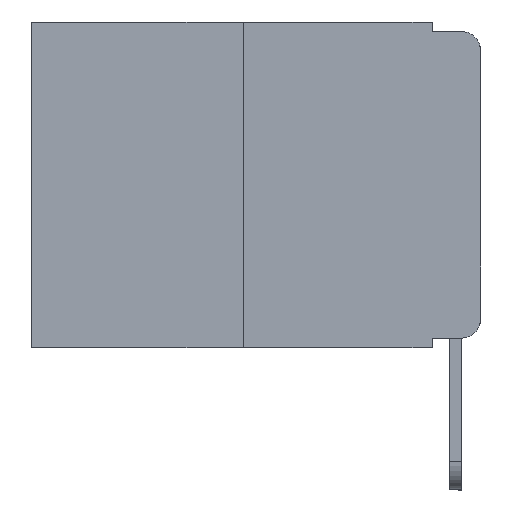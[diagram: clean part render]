
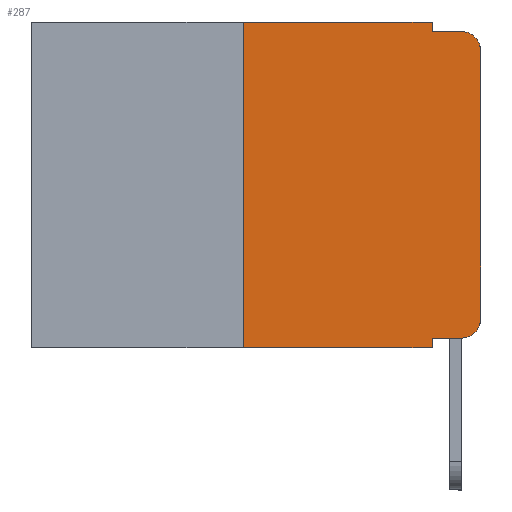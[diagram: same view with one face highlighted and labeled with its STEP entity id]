
A CAD part, left-side view. The second image highlights one B-rep face of the part: STEP entity #287.
In plain terms, the highlighted planar face has unit normal (-1, 0, 0).
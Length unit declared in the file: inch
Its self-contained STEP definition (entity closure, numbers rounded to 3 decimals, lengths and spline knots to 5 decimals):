
#204 = EDGE_CURVE ( 'NONE', #2949, #7871, #11588, .T. ) ;
#226 = VERTEX_POINT ( 'NONE', #18269 ) ;
#287 = ADVANCED_FACE ( 'NONE', ( #17137 ), #6791, .F. ) ;
#504 = ORIENTED_EDGE ( 'NONE', *, *, #10203, .T. ) ;
#596 = DIRECTION ( 'NONE',  ( -1., 0., 0. ) ) ;
#1010 = LINE ( 'NONE', #10817, #20700 ) ;
#1974 = EDGE_CURVE ( 'NONE', #20083, #2949, #19958, .T. ) ;
#2082 = EDGE_CURVE ( 'NONE', #226, #15848, #7178, .T. ) ;
#2559 = CARTESIAN_POINT ( 'NONE',  ( 0., 0.25, 0. ) ) ;
#2949 = VERTEX_POINT ( 'NONE', #16776 ) ;
#3070 = LINE ( 'NONE', #10297, #5269 ) ;
#3171 = DIRECTION ( 'NONE',  ( 0., -1., 0. ) ) ;
#3286 = EDGE_CURVE ( 'NONE', #4948, #20257, #3070, .T. ) ;
#3670 = CIRCLE ( 'NONE', #20002, 0.02 ) ;
#4026 = DIRECTION ( 'NONE',  ( 0., -1., 0. ) ) ;
#4035 = VECTOR ( 'NONE', #14112, 39.37008 ) ;
#4695 = CARTESIAN_POINT ( 'NONE',  ( 0., 0., -0.313 ) ) ;
#4697 = ORIENTED_EDGE ( 'NONE', *, *, #9662, .F. ) ;
#4778 = ORIENTED_EDGE ( 'NONE', *, *, #204, .F. ) ;
#4795 = EDGE_CURVE ( 'NONE', #19974, #226, #14518, .T. ) ;
#4948 = VERTEX_POINT ( 'NONE', #18631 ) ;
#4962 = VECTOR ( 'NONE', #15035, 39.37008 ) ;
#5269 = VECTOR ( 'NONE', #16875, 39.37008 ) ;
#5308 = DIRECTION ( 'NONE',  ( -1., 0., 0. ) ) ;
#6047 = CARTESIAN_POINT ( 'NONE',  ( 0., 0., 0. ) ) ;
#6791 = PLANE ( 'NONE',  #11714 ) ;
#6839 = ORIENTED_EDGE ( 'NONE', *, *, #1974, .F. ) ;
#7023 = VERTEX_POINT ( 'NONE', #7986 ) ;
#7178 = CIRCLE ( 'NONE', #19595, 0.02 ) ;
#7370 = ORIENTED_EDGE ( 'NONE', *, *, #10370, .T. ) ;
#7871 = VERTEX_POINT ( 'NONE', #12731 ) ;
#7986 = CARTESIAN_POINT ( 'NONE',  ( 0., 0.25, -0.343 ) ) ;
#8471 = DIRECTION ( 'NONE',  ( 1., 0., 0. ) ) ;
#9662 = EDGE_CURVE ( 'NONE', #7023, #20083, #17819, .T. ) ;
#9742 = ORIENTED_EDGE ( 'NONE', *, *, #9972, .F. ) ;
#9972 = EDGE_CURVE ( 'NONE', #7871, #15848, #1010, .T. ) ;
#10203 = EDGE_CURVE ( 'NONE', #20768, #19974, #3670, .T. ) ;
#10293 = CARTESIAN_POINT ( 'NONE',  ( 0., 0.02, -0.03 ) ) ;
#10297 = CARTESIAN_POINT ( 'NONE',  ( 0., 0.051, 0. ) ) ;
#10370 = EDGE_CURVE ( 'NONE', #7023, #20257, #12221, .T. ) ;
#10817 = CARTESIAN_POINT ( 'NONE',  ( 0., 0.051, -0.01 ) ) ;
#11588 = LINE ( 'NONE', #18483, #4962 ) ;
#11714 = AXIS2_PLACEMENT_3D ( 'NONE', #19130, #8471, #14023 ) ;
#11982 = DIRECTION ( 'NONE',  ( 0., 0., -1. ) ) ;
#12221 = LINE ( 'NONE', #15659, #4035 ) ;
#12380 = CARTESIAN_POINT ( 'NONE',  ( 0., 0.25, 0. ) ) ;
#12553 = VECTOR ( 'NONE', #16152, 39.37008 ) ;
#12731 = CARTESIAN_POINT ( 'NONE',  ( 0., 0.051, -0.01 ) ) ;
#13058 = ORIENTED_EDGE ( 'NONE', *, *, #4795, .T. ) ;
#13373 = CARTESIAN_POINT ( 'NONE',  ( 0., 0.02, -0.313 ) ) ;
#14023 = DIRECTION ( 'NONE',  ( 0., 0., -1. ) ) ;
#14112 = DIRECTION ( 'NONE',  ( 0., -1., 0. ) ) ;
#14518 = LINE ( 'NONE', #6047, #15546 ) ;
#15035 = DIRECTION ( 'NONE',  ( 0., 0., -1. ) ) ;
#15419 = DIRECTION ( 'NONE',  ( 0., -1., 0. ) ) ;
#15546 = VECTOR ( 'NONE', #19615, 39.37008 ) ;
#15659 = CARTESIAN_POINT ( 'NONE',  ( 0., 0.473, -0.343 ) ) ;
#15848 = VERTEX_POINT ( 'NONE', #20930 ) ;
#16038 = ORIENTED_EDGE ( 'NONE', *, *, #3286, .F. ) ;
#16058 = VECTOR ( 'NONE', #3171, 39.37008 ) ;
#16152 = DIRECTION ( 'NONE',  ( 0., 0., 1. ) ) ;
#16776 = CARTESIAN_POINT ( 'NONE',  ( 0., 0.051, 0. ) ) ;
#16779 = CARTESIAN_POINT ( 'NONE',  ( 0., 0.02, -0.333 ) ) ;
#16875 = DIRECTION ( 'NONE',  ( 0., 0., -1. ) ) ;
#17137 = FACE_OUTER_BOUND ( 'NONE', #20873, .T. ) ;
#17224 = DIRECTION ( 'NONE',  ( 0., 0., -1. ) ) ;
#17505 = ORIENTED_EDGE ( 'NONE', *, *, #2082, .T. ) ;
#17819 = LINE ( 'NONE', #2559, #12553 ) ;
#18269 = CARTESIAN_POINT ( 'NONE',  ( 0., 0., -0.03 ) ) ;
#18483 = CARTESIAN_POINT ( 'NONE',  ( 0., 0.051, 0. ) ) ;
#18631 = CARTESIAN_POINT ( 'NONE',  ( 0., 0.051, -0.333 ) ) ;
#18650 = CARTESIAN_POINT ( 'NONE',  ( 0., 0.473, 0. ) ) ;
#18979 = VECTOR ( 'NONE', #15419, 39.37008 ) ;
#19130 = CARTESIAN_POINT ( 'NONE',  ( 0., 0.473, 0. ) ) ;
#19561 = EDGE_CURVE ( 'NONE', #4948, #20768, #20076, .T. ) ;
#19595 = AXIS2_PLACEMENT_3D ( 'NONE', #10293, #596, #11982 ) ;
#19615 = DIRECTION ( 'NONE',  ( 0., 0., 1. ) ) ;
#19657 = ORIENTED_EDGE ( 'NONE', *, *, #19561, .T. ) ;
#19957 = CARTESIAN_POINT ( 'NONE',  ( 0., 0.051, -0.333 ) ) ;
#19958 = LINE ( 'NONE', #18650, #16058 ) ;
#19974 = VERTEX_POINT ( 'NONE', #4695 ) ;
#20002 = AXIS2_PLACEMENT_3D ( 'NONE', #13373, #5308, #17224 ) ;
#20076 = LINE ( 'NONE', #19957, #18979 ) ;
#20083 = VERTEX_POINT ( 'NONE', #12380 ) ;
#20257 = VERTEX_POINT ( 'NONE', #21146 ) ;
#20700 = VECTOR ( 'NONE', #4026, 39.37008 ) ;
#20768 = VERTEX_POINT ( 'NONE', #16779 ) ;
#20873 = EDGE_LOOP ( 'NONE', ( #13058, #17505, #9742, #4778, #6839, #4697, #7370, #16038, #19657, #504 ) ) ;
#20930 = CARTESIAN_POINT ( 'NONE',  ( 0., 0.02, -0.01 ) ) ;
#21146 = CARTESIAN_POINT ( 'NONE',  ( 0., 0.051, -0.343 ) ) ;
